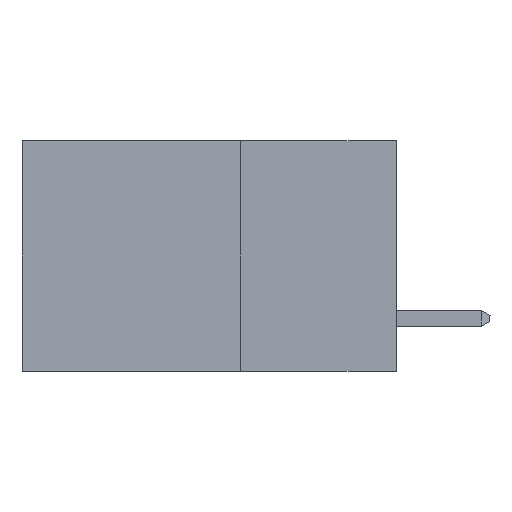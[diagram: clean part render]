
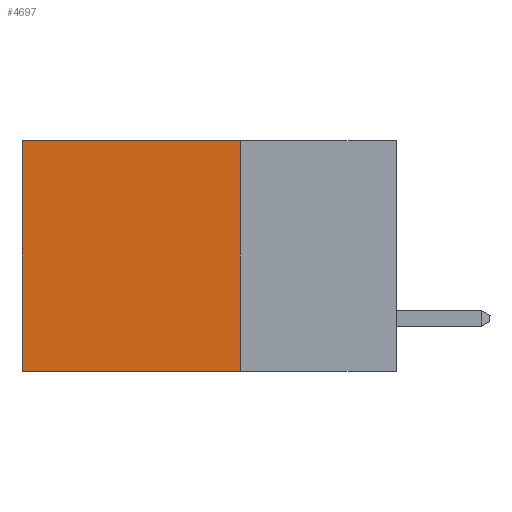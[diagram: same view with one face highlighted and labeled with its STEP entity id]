
A CAD part, left-side view. The second image highlights one B-rep face of the part: STEP entity #4697.
In plain terms, the highlighted planar face has unit normal (-1, 0, 0).
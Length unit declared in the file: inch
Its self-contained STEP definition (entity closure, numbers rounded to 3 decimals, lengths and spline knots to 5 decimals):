
#26 = VERTEX_POINT ( 'NONE', #5451 ) ;
#234 = VERTEX_POINT ( 'NONE', #16300 ) ;
#978 = CARTESIAN_POINT ( 'NONE',  ( 0.298, 0.6, 0. ) ) ;
#2737 = DIRECTION ( 'NONE',  ( 0., 0., -1. ) ) ;
#2743 = VECTOR ( 'NONE', #24641, 39.37008 ) ;
#4015 = AXIS2_PLACEMENT_3D ( 'NONE', #24755, #17128, #19080 ) ;
#4697 = ADVANCED_FACE ( 'NONE', ( #18094 ), #13417, .F. ) ;
#5451 = CARTESIAN_POINT ( 'NONE',  ( 0.298, 0.6, -0.37 ) ) ;
#6416 = EDGE_CURVE ( 'NONE', #23533, #26, #17094, .T. ) ;
#6713 = EDGE_CURVE ( 'NONE', #14465, #234, #14110, .T. ) ;
#7895 = LINE ( 'NONE', #11094, #2743 ) ;
#8795 = DIRECTION ( 'NONE',  ( 0., 0., -1. ) ) ;
#9319 = ORIENTED_EDGE ( 'NONE', *, *, #19945, .T. ) ;
#10027 = DIRECTION ( 'NONE',  ( 0., 1., 0. ) ) ;
#11094 = CARTESIAN_POINT ( 'NONE',  ( 0.298, 0.25, -0.37 ) ) ;
#12064 = CARTESIAN_POINT ( 'NONE',  ( 0.298, 0.25, 0. ) ) ;
#12304 = CARTESIAN_POINT ( 'NONE',  ( 0.298, 0.25, 0. ) ) ;
#13417 = PLANE ( 'NONE',  #4015 ) ;
#14110 = LINE ( 'NONE', #17786, #17397 ) ;
#14465 = VERTEX_POINT ( 'NONE', #12304 ) ;
#15334 = EDGE_LOOP ( 'NONE', ( #17145, #20655, #23038, #9319 ) ) ;
#16300 = CARTESIAN_POINT ( 'NONE',  ( 0.298, 0.25, -0.37 ) ) ;
#17094 = LINE ( 'NONE', #978, #18030 ) ;
#17128 = DIRECTION ( 'NONE',  ( 1., 0., 0. ) ) ;
#17145 = ORIENTED_EDGE ( 'NONE', *, *, #6416, .T. ) ;
#17359 = EDGE_CURVE ( 'NONE', #234, #26, #7895, .T. ) ;
#17397 = VECTOR ( 'NONE', #2737, 39.37008 ) ;
#17786 = CARTESIAN_POINT ( 'NONE',  ( 0.298, 0.25, 0. ) ) ;
#18030 = VECTOR ( 'NONE', #8795, 39.37008 ) ;
#18094 = FACE_OUTER_BOUND ( 'NONE', #15334, .T. ) ;
#19080 = DIRECTION ( 'NONE',  ( 0., 0., -1. ) ) ;
#19945 = EDGE_CURVE ( 'NONE', #14465, #23533, #24361, .T. ) ;
#20655 = ORIENTED_EDGE ( 'NONE', *, *, #17359, .F. ) ;
#21289 = VECTOR ( 'NONE', #10027, 39.37008 ) ;
#22365 = CARTESIAN_POINT ( 'NONE',  ( 0.298, 0.6, 0. ) ) ;
#23038 = ORIENTED_EDGE ( 'NONE', *, *, #6713, .F. ) ;
#23533 = VERTEX_POINT ( 'NONE', #22365 ) ;
#24361 = LINE ( 'NONE', #12064, #21289 ) ;
#24641 = DIRECTION ( 'NONE',  ( 0., 1., 0. ) ) ;
#24755 = CARTESIAN_POINT ( 'NONE',  ( 0.298, 0.25, 0. ) ) ;
